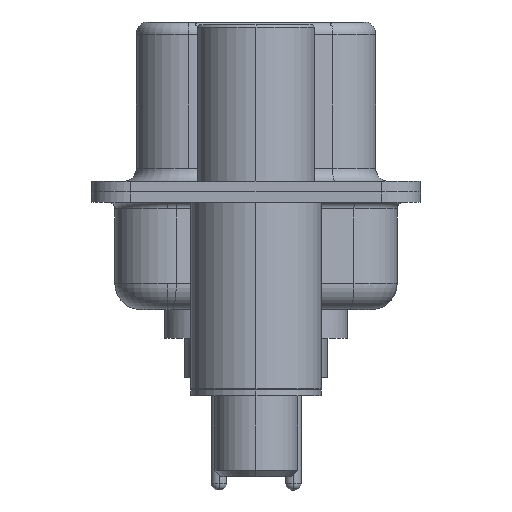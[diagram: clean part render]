
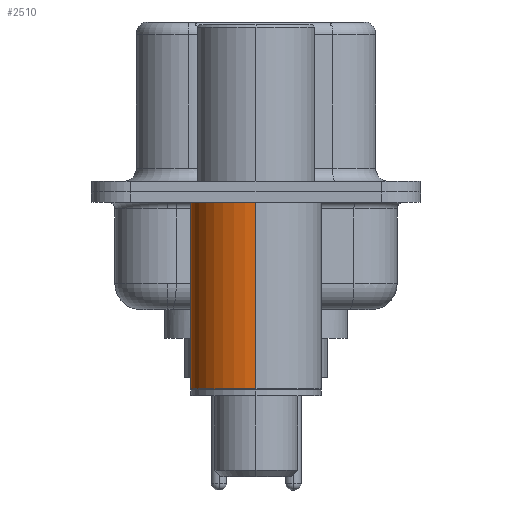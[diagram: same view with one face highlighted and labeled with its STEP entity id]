
A CAD part, left-side view. The second image highlights one B-rep face of the part: STEP entity #2510.
In plain terms, the highlighted cylindrical face has radius 2.5 mm (diameter 5 mm), a partial arc.
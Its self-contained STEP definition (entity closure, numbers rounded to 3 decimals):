
#237 = LINE ( 'NONE', #22040, #12606 ) ;
#391 = DIRECTION ( 'NONE',  ( 0., 0., 1. ) ) ;
#591 = DIRECTION ( 'NONE',  ( 0., 0., 1. ) ) ;
#1569 = VERTEX_POINT ( 'NONE', #13513 ) ;
#1586 = DIRECTION ( 'NONE',  ( 1., 0., 0. ) ) ;
#1936 = DIRECTION ( 'NONE',  ( 0., 0., 1. ) ) ;
#2510 = ADVANCED_FACE ( 'NONE', ( #11192 ), #27428, .T. ) ;
#2634 = AXIS2_PLACEMENT_3D ( 'NONE', #7305, #391, #3903 ) ;
#2951 = EDGE_CURVE ( 'NONE', #6578, #12057, #10397, .T. ) ;
#3903 = DIRECTION ( 'NONE',  ( 1., 0., 0. ) ) ;
#4236 = EDGE_CURVE ( 'NONE', #6578, #1569, #14042, .T. ) ;
#4909 = CARTESIAN_POINT ( 'NONE',  ( 2.5, 0., -7.525 ) ) ;
#6578 = VERTEX_POINT ( 'NONE', #4909 ) ;
#6646 = DIRECTION ( 'NONE',  ( 0., 0., 1. ) ) ;
#7305 = CARTESIAN_POINT ( 'NONE',  ( 0., 0., -7.525 ) ) ;
#7600 = VECTOR ( 'NONE', #15650, 1000. ) ;
#8175 = AXIS2_PLACEMENT_3D ( 'NONE', #14379, #1936, #1586 ) ;
#10397 = CIRCLE ( 'NONE', #2634, 2.5 ) ;
#11192 = FACE_OUTER_BOUND ( 'NONE', #19532, .T. ) ;
#11734 = ORIENTED_EDGE ( 'NONE', *, *, #23203, .T. ) ;
#12057 = VERTEX_POINT ( 'NONE', #26808 ) ;
#12606 = VECTOR ( 'NONE', #6646, 1000. ) ;
#12624 = CARTESIAN_POINT ( 'NONE',  ( 2.5, 0., 0.581 ) ) ;
#13513 = CARTESIAN_POINT ( 'NONE',  ( 2.5, 0., -0.4 ) ) ;
#13733 = CARTESIAN_POINT ( 'NONE',  ( 0., 0., -0.4 ) ) ;
#14042 = LINE ( 'NONE', #12624, #7600 ) ;
#14379 = CARTESIAN_POINT ( 'NONE',  ( 0., 0., 0.581 ) ) ;
#14987 = AXIS2_PLACEMENT_3D ( 'NONE', #13733, #591, #15939 ) ;
#15650 = DIRECTION ( 'NONE',  ( 0., 0., 1. ) ) ;
#15939 = DIRECTION ( 'NONE',  ( 1., 0., 0. ) ) ;
#16149 = ORIENTED_EDGE ( 'NONE', *, *, #2951, .T. ) ;
#16963 = CARTESIAN_POINT ( 'NONE',  ( -2.5, 0., -0.4 ) ) ;
#19532 = EDGE_LOOP ( 'NONE', ( #16149, #11734, #24503, #27162 ) ) ;
#21640 = CIRCLE ( 'NONE', #14987, 2.5 ) ;
#22040 = CARTESIAN_POINT ( 'NONE',  ( -2.5, 0., 0.581 ) ) ;
#23203 = EDGE_CURVE ( 'NONE', #12057, #23746, #237, .T. ) ;
#23746 = VERTEX_POINT ( 'NONE', #16963 ) ;
#24503 = ORIENTED_EDGE ( 'NONE', *, *, #27585, .F. ) ;
#26808 = CARTESIAN_POINT ( 'NONE',  ( -2.5, 0., -7.525 ) ) ;
#27162 = ORIENTED_EDGE ( 'NONE', *, *, #4236, .F. ) ;
#27428 = CYLINDRICAL_SURFACE ( 'NONE', #8175, 2.5 ) ;
#27585 = EDGE_CURVE ( 'NONE', #1569, #23746, #21640, .T. ) ;
